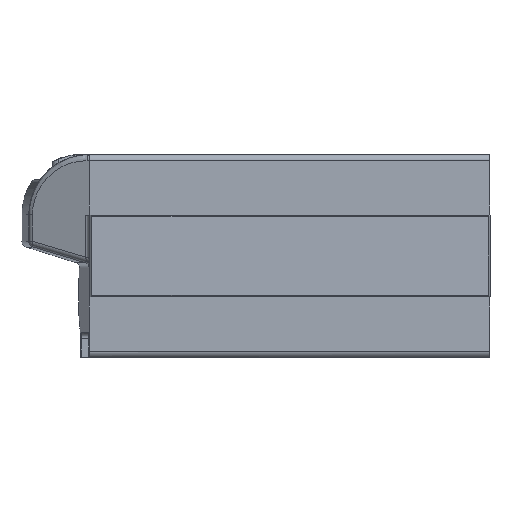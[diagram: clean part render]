
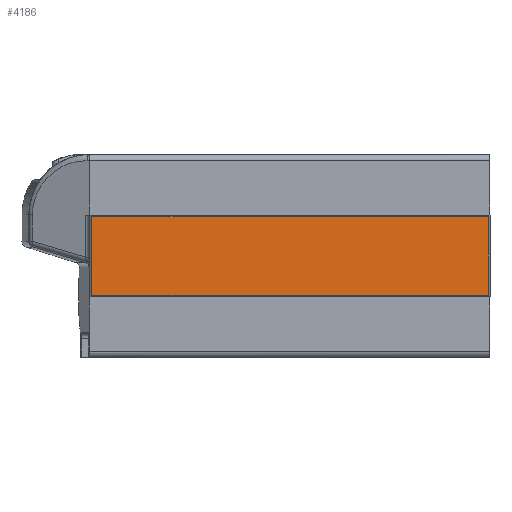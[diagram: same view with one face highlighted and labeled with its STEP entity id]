
A CAD part, left-side view. The second image highlights one B-rep face of the part: STEP entity #4186.
In plain terms, the highlighted planar face has unit normal (-1, -0.029, 0).
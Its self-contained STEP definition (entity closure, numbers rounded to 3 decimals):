
#2997 = VERTEX_POINT('',#2998);
#2998 = CARTESIAN_POINT('',(-28.4,-30.342,
    -3.246));
#3003 = EDGE_CURVE('',#3004,#2997,#3006,.T.);
#3004 = VERTEX_POINT('',#3005);
#3005 = CARTESIAN_POINT('',(-29.37,2.592,
    -3.246));
#3006 = LINE('',#3007,#3008);
#3007 = CARTESIAN_POINT('',(-29.416,4.134,
    -3.246));
#3008 = VECTOR('',#3009,1.);
#3009 = DIRECTION('',(0.029,-1.,0.));
#3090 = VERTEX_POINT('',#3091);
#3091 = CARTESIAN_POINT('',(-29.37,2.592,
    3.246));
#3096 = EDGE_CURVE('',#3090,#3097,#3099,.T.);
#3097 = VERTEX_POINT('',#3098);
#3098 = CARTESIAN_POINT('',(-28.4,-30.342,
    3.246));
#3099 = LINE('',#3100,#3101);
#3100 = CARTESIAN_POINT('',(-29.416,4.134,
    3.246));
#3101 = VECTOR('',#3102,1.);
#3102 = DIRECTION('',(0.029,-1.,0.));
#3120 = EDGE_CURVE('',#3090,#3004,#3121,.T.);
#3121 = LINE('',#3122,#3123);
#3122 = CARTESIAN_POINT('',(-29.37,2.592,8.425));
#3123 = VECTOR('',#3124,1.);
#3124 = DIRECTION('',(0.,0.,-1.));
#4175 = EDGE_CURVE('',#3097,#2997,#4176,.T.);
#4176 = LINE('',#4177,#4178);
#4177 = CARTESIAN_POINT('',(-28.4,-30.342,-8.425));
#4178 = VECTOR('',#4179,1.);
#4179 = DIRECTION('',(0.,0.,-1.));
#4186 = ADVANCED_FACE('',(#4187),#4193,.T.);
#4187 = FACE_BOUND('',#4188,.T.);
#4188 = EDGE_LOOP('',(#4189,#4190,#4191,#4192));
#4189 = ORIENTED_EDGE('',*,*,#3096,.F.);
#4190 = ORIENTED_EDGE('',*,*,#3120,.T.);
#4191 = ORIENTED_EDGE('',*,*,#3003,.T.);
#4192 = ORIENTED_EDGE('',*,*,#4175,.F.);
#4193 = PLANE('',#4194);
#4194 = AXIS2_PLACEMENT_3D('',#4195,#4196,#4197);
#4195 = CARTESIAN_POINT('',(-29.37,2.592,
    3.246));
#4196 = DIRECTION('',(-1.,-0.029,0.));
#4197 = DIRECTION('',(0.029,-0.981,-0.193
    ));
